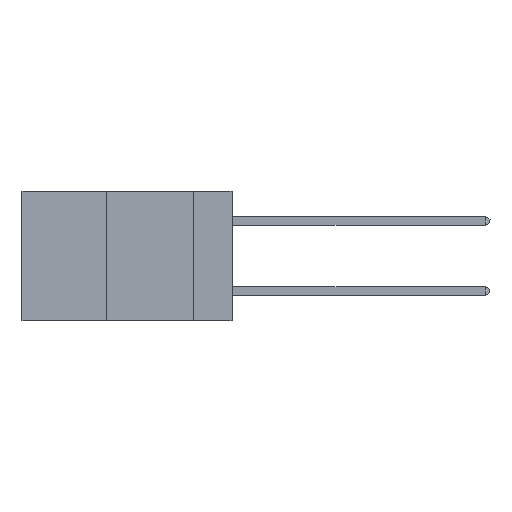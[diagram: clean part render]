
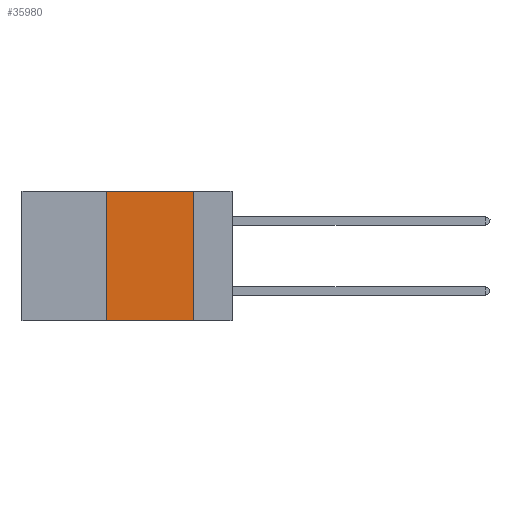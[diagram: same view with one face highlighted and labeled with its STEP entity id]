
A CAD part, left-side view. The second image highlights one B-rep face of the part: STEP entity #35980.
In plain terms, the highlighted planar face has unit normal (-1, 0, 0).
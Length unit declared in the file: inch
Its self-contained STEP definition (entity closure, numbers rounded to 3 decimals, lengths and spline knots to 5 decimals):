
#1761 = ORIENTED_EDGE ( 'NONE', *, *, #34322, .T. ) ;
#3233 = CARTESIAN_POINT ( 'NONE',  ( 0., 0.11, -0.37 ) ) ;
#3352 = CARTESIAN_POINT ( 'NONE',  ( 0., 0.36, -0.37 ) ) ;
#4808 = ORIENTED_EDGE ( 'NONE', *, *, #9674, .F. ) ;
#5519 = CARTESIAN_POINT ( 'NONE',  ( 0., 0.6, 0. ) ) ;
#6078 = LINE ( 'NONE', #19209, #42091 ) ;
#6145 = CARTESIAN_POINT ( 'NONE',  ( 0., 0.11, 0. ) ) ;
#8345 = AXIS2_PLACEMENT_3D ( 'NONE', #5519, #12010, #25122 ) ;
#9674 = EDGE_CURVE ( 'NONE', #36068, #12588, #6078, .T. ) ;
#9912 = CARTESIAN_POINT ( 'NONE',  ( 0., 0.36, 0. ) ) ;
#12010 = DIRECTION ( 'NONE',  ( 1., 0., 0. ) ) ;
#12588 = VERTEX_POINT ( 'NONE', #9912 ) ;
#12727 = EDGE_LOOP ( 'NONE', ( #14724, #25845, #4808, #1761 ) ) ;
#12764 = DIRECTION ( 'NONE',  ( 0., 0., -1. ) ) ;
#14724 = ORIENTED_EDGE ( 'NONE', *, *, #27499, .F. ) ;
#19209 = CARTESIAN_POINT ( 'NONE',  ( 0., 0.36, 0. ) ) ;
#19418 = CARTESIAN_POINT ( 'NONE',  ( 0., 0.11, 0. ) ) ;
#20101 = EDGE_CURVE ( 'NONE', #12588, #40256, #40745, .T. ) ;
#22510 = VERTEX_POINT ( 'NONE', #3233 ) ;
#24421 = VECTOR ( 'NONE', #39081, 39.37008 ) ;
#25122 = DIRECTION ( 'NONE',  ( 0., 0., -1. ) ) ;
#25845 = ORIENTED_EDGE ( 'NONE', *, *, #20101, .F. ) ;
#26167 = VECTOR ( 'NONE', #12764, 39.37008 ) ;
#27499 = EDGE_CURVE ( 'NONE', #40256, #22510, #42206, .T. ) ;
#27596 = VECTOR ( 'NONE', #40108, 39.37008 ) ;
#30653 = CARTESIAN_POINT ( 'NONE',  ( 0., 0.6, 0. ) ) ;
#32434 = CARTESIAN_POINT ( 'NONE',  ( 0., 0.6, -0.37 ) ) ;
#32845 = LINE ( 'NONE', #32434, #24421 ) ;
#34322 = EDGE_CURVE ( 'NONE', #36068, #22510, #32845, .T. ) ;
#34986 = PLANE ( 'NONE',  #8345 ) ;
#35752 = DIRECTION ( 'NONE',  ( 0., 0., 1. ) ) ;
#35980 = ADVANCED_FACE ( 'NONE', ( #38199 ), #34986, .F. ) ;
#36068 = VERTEX_POINT ( 'NONE', #3352 ) ;
#38199 = FACE_OUTER_BOUND ( 'NONE', #12727, .T. ) ;
#39081 = DIRECTION ( 'NONE',  ( 0., -1., 0. ) ) ;
#40108 = DIRECTION ( 'NONE',  ( 0., -1., 0. ) ) ;
#40256 = VERTEX_POINT ( 'NONE', #6145 ) ;
#40745 = LINE ( 'NONE', #30653, #27596 ) ;
#42091 = VECTOR ( 'NONE', #35752, 39.37008 ) ;
#42206 = LINE ( 'NONE', #19418, #26167 ) ;
